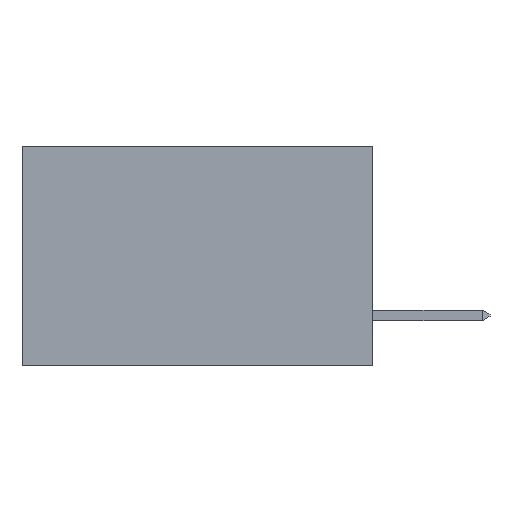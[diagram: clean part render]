
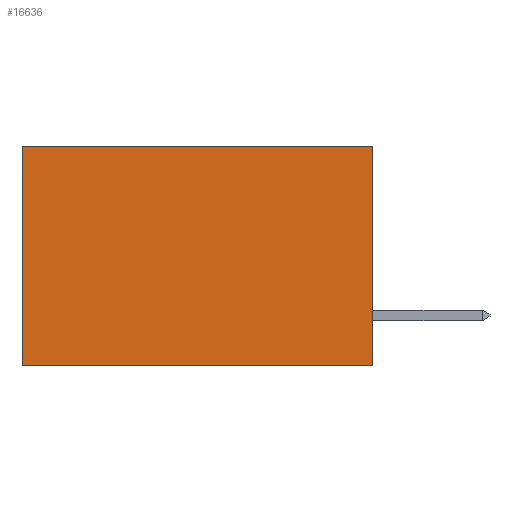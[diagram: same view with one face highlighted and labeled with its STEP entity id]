
A CAD part, left-side view. The second image highlights one B-rep face of the part: STEP entity #16636.
In plain terms, the highlighted planar face has unit normal (-1, 0, 0).
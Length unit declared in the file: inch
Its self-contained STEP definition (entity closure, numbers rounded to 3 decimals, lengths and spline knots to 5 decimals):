
#331 = ORIENTED_EDGE ( 'NONE', *, *, #3776, .F. ) ;
#843 = CARTESIAN_POINT ( 'NONE',  ( 0.277, 0., -0.37 ) ) ;
#1201 = VECTOR ( 'NONE', #7329, 39.37008 ) ;
#2120 = DIRECTION ( 'NONE',  ( 1., 0., 0. ) ) ;
#3687 = PLANE ( 'NONE',  #14460 ) ;
#3776 = EDGE_CURVE ( 'NONE', #16410, #17766, #5344, .T. ) ;
#4491 = FACE_OUTER_BOUND ( 'NONE', #20498, .T. ) ;
#4561 = CARTESIAN_POINT ( 'NONE',  ( 0.277, 0., 0. ) ) ;
#4823 = VECTOR ( 'NONE', #13587, 39.37008 ) ;
#4850 = ORIENTED_EDGE ( 'NONE', *, *, #20914, .T. ) ;
#5344 = LINE ( 'NONE', #18089, #4823 ) ;
#7329 = DIRECTION ( 'NONE',  ( 0., 0., -1. ) ) ;
#9380 = VERTEX_POINT ( 'NONE', #10566 ) ;
#9613 = CARTESIAN_POINT ( 'NONE',  ( 0.277, 0.59, -0.37 ) ) ;
#9790 = VECTOR ( 'NONE', #14299, 39.37008 ) ;
#10566 = CARTESIAN_POINT ( 'NONE',  ( 0.277, 0.59, 0. ) ) ;
#11811 = CARTESIAN_POINT ( 'NONE',  ( 0.277, 0., -0.37 ) ) ;
#12086 = EDGE_CURVE ( 'NONE', #9380, #17766, #18624, .T. ) ;
#13455 = DIRECTION ( 'NONE',  ( 0., 0., -1. ) ) ;
#13587 = DIRECTION ( 'NONE',  ( 0., 1., 0. ) ) ;
#13754 = VECTOR ( 'NONE', #19324, 39.37008 ) ;
#13883 = ORIENTED_EDGE ( 'NONE', *, *, #12086, .T. ) ;
#14299 = DIRECTION ( 'NONE',  ( 0., 1., 0. ) ) ;
#14460 = AXIS2_PLACEMENT_3D ( 'NONE', #11811, #2120, #13455 ) ;
#14560 = CARTESIAN_POINT ( 'NONE',  ( 0.277, 0., -0.37 ) ) ;
#15503 = CARTESIAN_POINT ( 'NONE',  ( 0.277, 0., 0. ) ) ;
#16153 = EDGE_CURVE ( 'NONE', #19435, #16410, #19011, .T. ) ;
#16410 = VERTEX_POINT ( 'NONE', #14560 ) ;
#16636 = ADVANCED_FACE ( 'NONE', ( #4491 ), #3687, .F. ) ;
#17464 = LINE ( 'NONE', #4561, #9790 ) ;
#17766 = VERTEX_POINT ( 'NONE', #9613 ) ;
#18089 = CARTESIAN_POINT ( 'NONE',  ( 0.277, 0., -0.37 ) ) ;
#18624 = LINE ( 'NONE', #20868, #13754 ) ;
#18787 = ORIENTED_EDGE ( 'NONE', *, *, #16153, .F. ) ;
#19011 = LINE ( 'NONE', #843, #1201 ) ;
#19324 = DIRECTION ( 'NONE',  ( 0., 0., -1. ) ) ;
#19435 = VERTEX_POINT ( 'NONE', #15503 ) ;
#20498 = EDGE_LOOP ( 'NONE', ( #13883, #331, #18787, #4850 ) ) ;
#20868 = CARTESIAN_POINT ( 'NONE',  ( 0.277, 0.59, -0.37 ) ) ;
#20914 = EDGE_CURVE ( 'NONE', #19435, #9380, #17464, .T. ) ;
